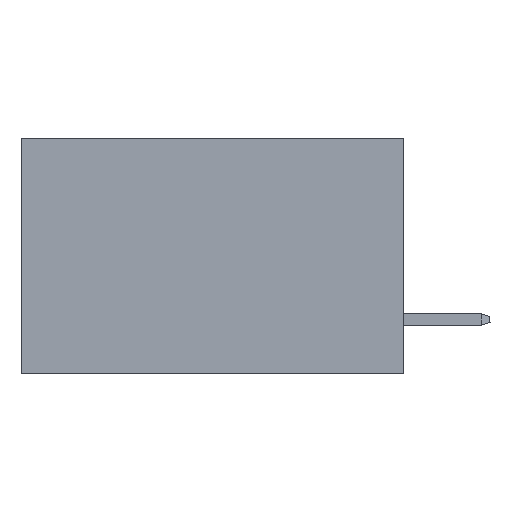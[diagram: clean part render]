
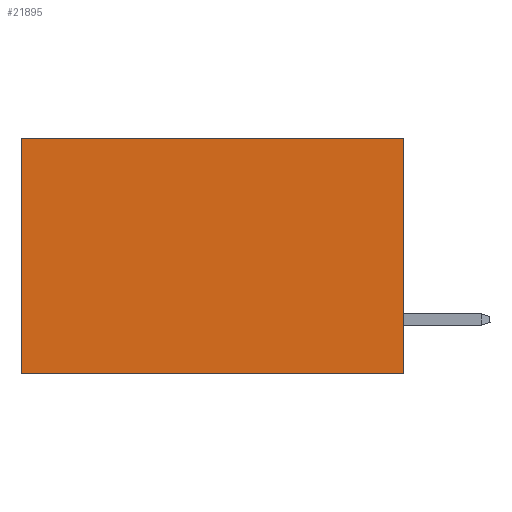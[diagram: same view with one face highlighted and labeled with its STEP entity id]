
A CAD part, left-side view. The second image highlights one B-rep face of the part: STEP entity #21895.
In plain terms, the highlighted planar face has unit normal (-1, 0, 0).
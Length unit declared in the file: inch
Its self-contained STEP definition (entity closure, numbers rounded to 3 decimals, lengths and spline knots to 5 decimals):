
#226 = DIRECTION ( 'NONE',  ( 0., 1., 0. ) ) ;
#613 = VERTEX_POINT ( 'NONE', #11341 ) ;
#2567 = ORIENTED_EDGE ( 'NONE', *, *, #30141, .F. ) ;
#2906 = VERTEX_POINT ( 'NONE', #5231 ) ;
#3191 = CARTESIAN_POINT ( 'NONE',  ( 0.2875, 0., -0.37 ) ) ;
#4132 = CARTESIAN_POINT ( 'NONE',  ( 0.2875, 0., 0. ) ) ;
#4404 = LINE ( 'NONE', #30625, #21165 ) ;
#5231 = CARTESIAN_POINT ( 'NONE',  ( 0.2875, 0., -0.37 ) ) ;
#5275 = ORIENTED_EDGE ( 'NONE', *, *, #31335, .T. ) ;
#6558 = LINE ( 'NONE', #4132, #12726 ) ;
#6675 = DIRECTION ( 'NONE',  ( 0., 1., 0. ) ) ;
#6841 = EDGE_CURVE ( 'NONE', #2906, #613, #24145, .T. ) ;
#7232 = ORIENTED_EDGE ( 'NONE', *, *, #30819, .T. ) ;
#7320 = VECTOR ( 'NONE', #226, 39.37008 ) ;
#8141 = CARTESIAN_POINT ( 'NONE',  ( 0.2875, 0.6, 0. ) ) ;
#8369 = VECTOR ( 'NONE', #10529, 39.37008 ) ;
#9566 = PLANE ( 'NONE',  #33482 ) ;
#10529 = DIRECTION ( 'NONE',  ( 0., 0., -1. ) ) ;
#11341 = CARTESIAN_POINT ( 'NONE',  ( 0.2875, 0.6, -0.37 ) ) ;
#11698 = ORIENTED_EDGE ( 'NONE', *, *, #6841, .F. ) ;
#12726 = VECTOR ( 'NONE', #27912, 39.37008 ) ;
#17777 = DIRECTION ( 'NONE',  ( 1., 0., 0. ) ) ;
#20225 = FACE_OUTER_BOUND ( 'NONE', #31905, .T. ) ;
#21053 = CARTESIAN_POINT ( 'NONE',  ( 0.2875, 0.6, 0. ) ) ;
#21165 = VECTOR ( 'NONE', #6675, 39.37008 ) ;
#21577 = LINE ( 'NONE', #8141, #8369 ) ;
#21895 = ADVANCED_FACE ( 'NONE', ( #20225 ), #9566, .F. ) ;
#23349 = CARTESIAN_POINT ( 'NONE',  ( 0.2875, 0., 0. ) ) ;
#23369 = VERTEX_POINT ( 'NONE', #21053 ) ;
#24145 = LINE ( 'NONE', #3191, #7320 ) ;
#25831 = DIRECTION ( 'NONE',  ( 0., 0., -1. ) ) ;
#27912 = DIRECTION ( 'NONE',  ( 0., 0., -1. ) ) ;
#30141 = EDGE_CURVE ( 'NONE', #34297, #2906, #6558, .T. ) ;
#30625 = CARTESIAN_POINT ( 'NONE',  ( 0.2875, 0., 0. ) ) ;
#30819 = EDGE_CURVE ( 'NONE', #34297, #23369, #4404, .T. ) ;
#31078 = CARTESIAN_POINT ( 'NONE',  ( 0.2875, 0., 0. ) ) ;
#31335 = EDGE_CURVE ( 'NONE', #23369, #613, #21577, .T. ) ;
#31905 = EDGE_LOOP ( 'NONE', ( #5275, #11698, #2567, #7232 ) ) ;
#33482 = AXIS2_PLACEMENT_3D ( 'NONE', #31078, #17777, #25831 ) ;
#34297 = VERTEX_POINT ( 'NONE', #23349 ) ;
